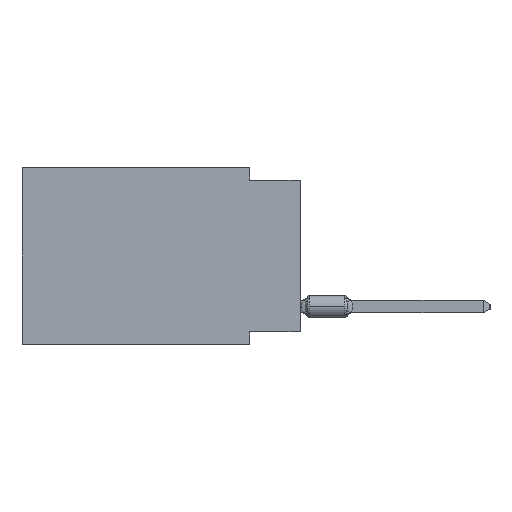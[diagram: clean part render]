
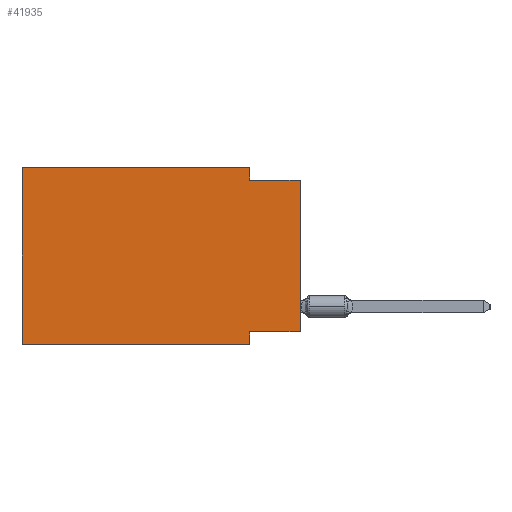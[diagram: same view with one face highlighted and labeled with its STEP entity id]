
A CAD part, left-side view. The second image highlights one B-rep face of the part: STEP entity #41935.
In plain terms, the highlighted planar face has unit normal (-1, 0, 0).
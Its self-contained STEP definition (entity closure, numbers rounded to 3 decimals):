
#2590 = LINE ( 'NONE', #44600, #29628 ) ;
#2656 = DIRECTION ( 'NONE',  ( 0., -1., 0. ) ) ;
#3705 = LINE ( 'NONE', #27876, #42772 ) ;
#6375 = VERTEX_POINT ( 'NONE', #8455 ) ;
#7346 = VECTOR ( 'NONE', #55564, 1000. ) ;
#7797 = EDGE_CURVE ( 'NONE', #12553, #6375, #45224, .T. ) ;
#8455 = CARTESIAN_POINT ( 'NONE',  ( 0., 2.54, -8.89 ) ) ;
#9805 = CARTESIAN_POINT ( 'NONE',  ( 0., 2.54, 0. ) ) ;
#11287 = DIRECTION ( 'NONE',  ( 0., 0., -1. ) ) ;
#11872 = CARTESIAN_POINT ( 'NONE',  ( 0., 0., 0. ) ) ;
#12259 = LINE ( 'NONE', #11872, #53535 ) ;
#12497 = EDGE_LOOP ( 'NONE', ( #75314, #17016, #72136, #66352, #70379, #35230, #68479, #50509 ) ) ;
#12553 = VERTEX_POINT ( 'NONE', #47153 ) ;
#14860 = DIRECTION ( 'NONE',  ( 0., -1., 0. ) ) ;
#17016 = ORIENTED_EDGE ( 'NONE', *, *, #33640, .F. ) ;
#19338 = VERTEX_POINT ( 'NONE', #48804 ) ;
#20044 = VERTEX_POINT ( 'NONE', #52250 ) ;
#20990 = EDGE_CURVE ( 'NONE', #12553, #20044, #2590, .T. ) ;
#21589 = VERTEX_POINT ( 'NONE', #51649 ) ;
#21926 = VECTOR ( 'NONE', #14860, 1000. ) ;
#26199 = AXIS2_PLACEMENT_3D ( 'NONE', #35666, #66993, #47174 ) ;
#27876 = CARTESIAN_POINT ( 'NONE',  ( 0., 2.54, -8.89 ) ) ;
#29628 = VECTOR ( 'NONE', #62850, 1000. ) ;
#31535 = LINE ( 'NONE', #56095, #21926 ) ;
#33640 = EDGE_CURVE ( 'NONE', #21589, #38638, #56961, .T. ) ;
#35078 = LINE ( 'NONE', #53319, #36370 ) ;
#35230 = ORIENTED_EDGE ( 'NONE', *, *, #7797, .T. ) ;
#35666 = CARTESIAN_POINT ( 'NONE',  ( 0., 13.97, 0. ) ) ;
#36370 = VECTOR ( 'NONE', #11287, 1000. ) ;
#36442 = DIRECTION ( 'NONE',  ( 0., 0., 1. ) ) ;
#38638 = VERTEX_POINT ( 'NONE', #63236 ) ;
#40910 = DIRECTION ( 'NONE',  ( 0., 0., -1. ) ) ;
#41046 = VECTOR ( 'NONE', #2656, 1000. ) ;
#41527 = VECTOR ( 'NONE', #43069, 1000. ) ;
#41935 = ADVANCED_FACE ( 'NONE', ( #65432 ), #54314, .F. ) ;
#42772 = VECTOR ( 'NONE', #40910, 1000. ) ;
#43069 = DIRECTION ( 'NONE',  ( 0., 1., 0. ) ) ;
#43124 = EDGE_CURVE ( 'NONE', #58352, #6375, #3705, .T. ) ;
#43465 = CARTESIAN_POINT ( 'NONE',  ( 0., 0., -8.255 ) ) ;
#43597 = EDGE_CURVE ( 'NONE', #19338, #58352, #49023, .T. ) ;
#43983 = EDGE_CURVE ( 'NONE', #54558, #21589, #35078, .T. ) ;
#44600 = CARTESIAN_POINT ( 'NONE',  ( 0., 13.97, 0. ) ) ;
#45224 = LINE ( 'NONE', #56330, #7346 ) ;
#47153 = CARTESIAN_POINT ( 'NONE',  ( 0., 13.97, -8.89 ) ) ;
#47174 = DIRECTION ( 'NONE',  ( 0., 0., -1. ) ) ;
#48804 = CARTESIAN_POINT ( 'NONE',  ( 0., 0., -8.255 ) ) ;
#49023 = LINE ( 'NONE', #43465, #41527 ) ;
#50509 = ORIENTED_EDGE ( 'NONE', *, *, #43597, .F. ) ;
#51649 = CARTESIAN_POINT ( 'NONE',  ( 0., 2.54, -0.635 ) ) ;
#52250 = CARTESIAN_POINT ( 'NONE',  ( 0., 13.97, 0. ) ) ;
#53319 = CARTESIAN_POINT ( 'NONE',  ( 0., 2.54, 0. ) ) ;
#53535 = VECTOR ( 'NONE', #36442, 1000. ) ;
#54314 = PLANE ( 'NONE',  #26199 ) ;
#54558 = VERTEX_POINT ( 'NONE', #9805 ) ;
#55564 = DIRECTION ( 'NONE',  ( 0., -1., 0. ) ) ;
#56095 = CARTESIAN_POINT ( 'NONE',  ( 0., 13.97, 0. ) ) ;
#56180 = CARTESIAN_POINT ( 'NONE',  ( 0., 0., -0.635 ) ) ;
#56330 = CARTESIAN_POINT ( 'NONE',  ( 0., 13.97, -8.89 ) ) ;
#56961 = LINE ( 'NONE', #56180, #41046 ) ;
#58352 = VERTEX_POINT ( 'NONE', #61937 ) ;
#60848 = EDGE_CURVE ( 'NONE', #20044, #54558, #31535, .T. ) ;
#61937 = CARTESIAN_POINT ( 'NONE',  ( 0., 2.54, -8.255 ) ) ;
#62850 = DIRECTION ( 'NONE',  ( 0., 0., 1. ) ) ;
#63236 = CARTESIAN_POINT ( 'NONE',  ( 0., 0., -0.635 ) ) ;
#65432 = FACE_OUTER_BOUND ( 'NONE', #12497, .T. ) ;
#66352 = ORIENTED_EDGE ( 'NONE', *, *, #60848, .F. ) ;
#66993 = DIRECTION ( 'NONE',  ( 1., 0., 0. ) ) ;
#68479 = ORIENTED_EDGE ( 'NONE', *, *, #43124, .F. ) ;
#70379 = ORIENTED_EDGE ( 'NONE', *, *, #20990, .F. ) ;
#72136 = ORIENTED_EDGE ( 'NONE', *, *, #43983, .F. ) ;
#73380 = EDGE_CURVE ( 'NONE', #19338, #38638, #12259, .T. ) ;
#75314 = ORIENTED_EDGE ( 'NONE', *, *, #73380, .T. ) ;
